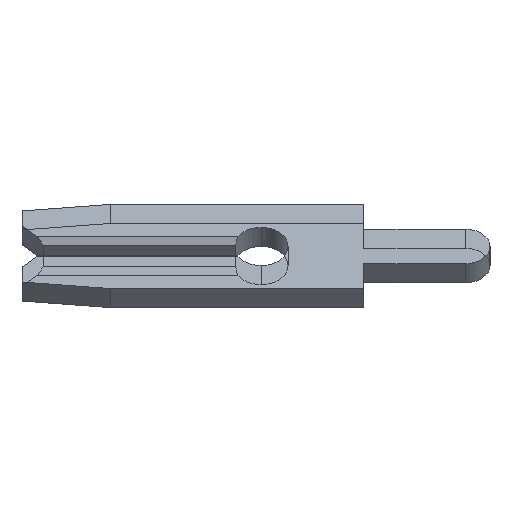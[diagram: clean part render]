
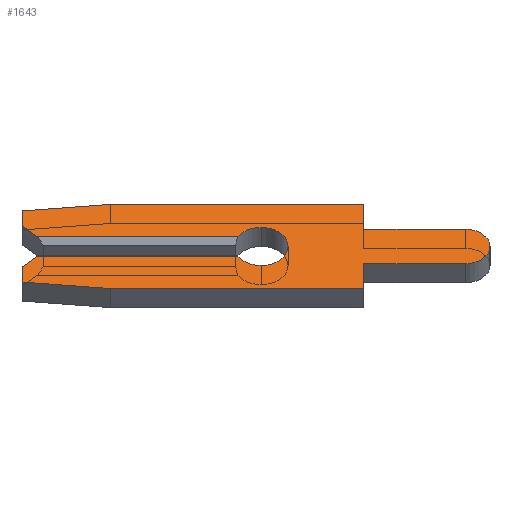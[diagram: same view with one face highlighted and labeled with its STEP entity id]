
A CAD part, left-side view. The second image highlights one B-rep face of the part: STEP entity #1643.
In plain terms, the highlighted face is planar.
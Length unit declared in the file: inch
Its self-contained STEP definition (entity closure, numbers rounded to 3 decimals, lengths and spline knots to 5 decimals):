
#25 = VERTEX_POINT ( 'NONE', #2202 ) ;
#42 = DIRECTION ( 'NONE',  ( 0., 0.995, 0.105 ) ) ;
#48 = CARTESIAN_POINT ( 'NONE',  ( -0.013, 0., 0. ) ) ;
#61 = LINE ( 'NONE', #1256, #2127 ) ;
#97 = FACE_OUTER_BOUND ( 'NONE', #2374, .T. ) ;
#131 = LINE ( 'NONE', #2694, #1034 ) ;
#137 = CARTESIAN_POINT ( 'NONE',  ( -0.013, 0.231, -0.028 ) ) ;
#149 = DIRECTION ( 'NONE',  ( 0., -1., 0. ) ) ;
#158 = CIRCLE ( 'NONE', #1631, 0.026 ) ;
#190 = VECTOR ( 'NONE', #2480, 39.37008 ) ;
#211 = DIRECTION ( 'NONE',  ( 0., 1., 0. ) ) ;
#214 = CARTESIAN_POINT ( 'NONE',  ( -0.013, 0.146, -0.0575 ) ) ;
#241 = DIRECTION ( 'NONE',  ( 0., 0., 1. ) ) ;
#283 = VERTEX_POINT ( 'NONE', #912 ) ;
#287 = ORIENTED_EDGE ( 'NONE', *, *, #1751, .T. ) ;
#288 = DIRECTION ( 'NONE',  ( -1., 0., 0. ) ) ;
#302 = VECTOR ( 'NONE', #211, 39.37008 ) ;
#349 = VERTEX_POINT ( 'NONE', #1965 ) ;
#353 = EDGE_CURVE ( 'NONE', #349, #859, #659, .T. ) ;
#354 = CARTESIAN_POINT ( 'NONE',  ( -0.013, 0.231, -0.04857 ) ) ;
#442 = VERTEX_POINT ( 'NONE', #2234 ) ;
#444 = ORIENTED_EDGE ( 'NONE', *, *, #353, .F. ) ;
#471 = AXIS2_PLACEMENT_3D ( 'NONE', #1158, #2653, #241 ) ;
#498 = DIRECTION ( 'NONE',  ( 0., 0., -1. ) ) ;
#543 = DIRECTION ( 'NONE',  ( 0., -0.707, 0.707 ) ) ;
#551 = LINE ( 'NONE', #764, #583 ) ;
#583 = VECTOR ( 'NONE', #543, 39.37008 ) ;
#588 = CARTESIAN_POINT ( 'NONE',  ( -0.013, -0.099, 0.0575 ) ) ;
#619 = VECTOR ( 'NONE', #1508, 39.37008 ) ;
#635 = DIRECTION ( 'NONE',  ( 0., 0., -1. ) ) ;
#645 = EDGE_CURVE ( 'NONE', #779, #1606, #2792, .T. ) ;
#659 = LINE ( 'NONE', #1589, #302 ) ;
#667 = LINE ( 'NONE', #137, #722 ) ;
#681 = EDGE_CURVE ( 'NONE', #1288, #2090, #131, .T. ) ;
#722 = VECTOR ( 'NONE', #1015, 39.37008 ) ;
#724 = ORIENTED_EDGE ( 'NONE', *, *, #2002, .F. ) ;
#764 = CARTESIAN_POINT ( 'NONE',  ( -0.013, 0.2105, -0.0075 ) ) ;
#769 = ORIENTED_EDGE ( 'NONE', *, *, #1484, .F. ) ;
#779 = VERTEX_POINT ( 'NONE', #214 ) ;
#782 = LINE ( 'NONE', #1839, #1663 ) ;
#784 = VECTOR ( 'NONE', #1238, 39.37008 ) ;
#800 = CARTESIAN_POINT ( 'NONE',  ( -0.013, 0.2105, 0.0075 ) ) ;
#839 = VERTEX_POINT ( 'NONE', #1217 ) ;
#841 = EDGE_CURVE ( 'NONE', #283, #2540, #1185, .T. ) ;
#859 = VERTEX_POINT ( 'NONE', #1626 ) ;
#865 = VERTEX_POINT ( 'NONE', #1412 ) ;
#892 = VECTOR ( 'NONE', #2773, 39.37008 ) ;
#912 = CARTESIAN_POINT ( 'NONE',  ( -0.013, 0.02252, -0.013 ) ) ;
#929 = LINE ( 'NONE', #2188, #1524 ) ;
#942 = ORIENTED_EDGE ( 'NONE', *, *, #1249, .F. ) ;
#1007 = CARTESIAN_POINT ( 'NONE',  ( -0.013, 0.146, 0.0575 ) ) ;
#1015 = DIRECTION ( 'NONE',  ( 0., 0., 1. ) ) ;
#1034 = VECTOR ( 'NONE', #1646, 39.37008 ) ;
#1036 = EDGE_CURVE ( 'NONE', #1885, #283, #2604, .T. ) ;
#1080 = ORIENTED_EDGE ( 'NONE', *, *, #645, .F. ) ;
#1108 = CIRCLE ( 'NONE', #1919, 0.026 ) ;
#1111 = VECTOR ( 'NONE', #42, 39.37008 ) ;
#1147 = LINE ( 'NONE', #1500, #619 ) ;
#1158 = CARTESIAN_POINT ( 'NONE',  ( -0.013, -0.1975, 0. ) ) ;
#1174 = CARTESIAN_POINT ( 'NONE',  ( -0.013, 0., 0. ) ) ;
#1185 = CIRCLE ( 'NONE', #1266, 0.026 ) ;
#1217 = CARTESIAN_POINT ( 'NONE',  ( -0.013, 0.146, 0.0575 ) ) ;
#1221 = LINE ( 'NONE', #1756, #190 ) ;
#1238 = DIRECTION ( 'NONE',  ( 0., -1., 0. ) ) ;
#1249 = EDGE_CURVE ( 'NONE', #865, #25, #1565, .T. ) ;
#1256 = CARTESIAN_POINT ( 'NONE',  ( -0.013, 0.146, -0.0575 ) ) ;
#1266 = AXIS2_PLACEMENT_3D ( 'NONE', #48, #288, #498 ) ;
#1288 = VERTEX_POINT ( 'NONE', #1461 ) ;
#1319 = VECTOR ( 'NONE', #2176, 39.37008 ) ;
#1341 = EDGE_CURVE ( 'NONE', #2473, #1885, #551, .T. ) ;
#1351 = ORIENTED_EDGE ( 'NONE', *, *, #1445, .F. ) ;
#1376 = CARTESIAN_POINT ( 'NONE',  ( -0.013, -0.1975, 0.0235 ) ) ;
#1398 = EDGE_CURVE ( 'NONE', #839, #2768, #2130, .T. ) ;
#1412 = CARTESIAN_POINT ( 'NONE',  ( -0.013, 0.231, 0.028 ) ) ;
#1423 = ORIENTED_EDGE ( 'NONE', *, *, #2588, .F. ) ;
#1445 = EDGE_CURVE ( 'NONE', #1606, #2473, #667, .T. ) ;
#1461 = CARTESIAN_POINT ( 'NONE',  ( -0.013, -0.099, 0.0235 ) ) ;
#1471 = ORIENTED_EDGE ( 'NONE', *, *, #2355, .F. ) ;
#1476 = CARTESIAN_POINT ( 'NONE',  ( -0.013, 0., 0. ) ) ;
#1484 = EDGE_CURVE ( 'NONE', #442, #779, #61, .T. ) ;
#1489 = CARTESIAN_POINT ( 'NONE',  ( -0.013, 0.02252, 0.013 ) ) ;
#1500 = CARTESIAN_POINT ( 'NONE',  ( -0.013, -0.099, -0.0575 ) ) ;
#1508 = DIRECTION ( 'NONE',  ( 0., 0., -1. ) ) ;
#1524 = VECTOR ( 'NONE', #149, 39.37008 ) ;
#1565 = LINE ( 'NONE', #2133, #2680 ) ;
#1589 = CARTESIAN_POINT ( 'NONE',  ( -0.013, -0.099, -0.0235 ) ) ;
#1603 = VERTEX_POINT ( 'NONE', #1489 ) ;
#1606 = VERTEX_POINT ( 'NONE', #354 ) ;
#1615 = CARTESIAN_POINT ( 'NONE',  ( -0.013, 0.231, -0.028 ) ) ;
#1622 = DIRECTION ( 'NONE',  ( 0., 0., -1. ) ) ;
#1626 = CARTESIAN_POINT ( 'NONE',  ( -0.013, -0.099, -0.0235 ) ) ;
#1631 = AXIS2_PLACEMENT_3D ( 'NONE', #1476, #2619, #2851 ) ;
#1635 = ORIENTED_EDGE ( 'NONE', *, *, #2047, .F. ) ;
#1638 = EDGE_CURVE ( 'NONE', #859, #442, #1147, .T. ) ;
#1643 = ADVANCED_FACE ( 'NONE', ( #97 ), #1949, .F. ) ;
#1646 = DIRECTION ( 'NONE',  ( 0., -1., 0. ) ) ;
#1663 = VECTOR ( 'NONE', #2432, 39.37008 ) ;
#1671 = ORIENTED_EDGE ( 'NONE', *, *, #1789, .F. ) ;
#1681 = DIRECTION ( 'NONE',  ( 0., 0., 1. ) ) ;
#1695 = DIRECTION ( 'NONE',  ( 0., 1., 0. ) ) ;
#1751 = EDGE_CURVE ( 'NONE', #2097, #1603, #929, .T. ) ;
#1756 = CARTESIAN_POINT ( 'NONE',  ( -0.013, -0.099, 0.0575 ) ) ;
#1759 = ORIENTED_EDGE ( 'NONE', *, *, #1992, .F. ) ;
#1789 = EDGE_CURVE ( 'NONE', #2031, #1603, #158, .T. ) ;
#1839 = CARTESIAN_POINT ( 'NONE',  ( -0.013, 0.231, 0.04857 ) ) ;
#1856 = ORIENTED_EDGE ( 'NONE', *, *, #1398, .F. ) ;
#1885 = VERTEX_POINT ( 'NONE', #2209 ) ;
#1919 = AXIS2_PLACEMENT_3D ( 'NONE', #1174, #2742, #1622 ) ;
#1949 = PLANE ( 'NONE',  #2478 ) ;
#1965 = CARTESIAN_POINT ( 'NONE',  ( -0.013, -0.1975, -0.0235 ) ) ;
#1972 = CARTESIAN_POINT ( 'NONE',  ( -0.013, 0., 0. ) ) ;
#1992 = EDGE_CURVE ( 'NONE', #25, #839, #782, .T. ) ;
#2002 = EDGE_CURVE ( 'NONE', #2768, #1288, #1221, .T. ) ;
#2028 = ORIENTED_EDGE ( 'NONE', *, *, #1341, .F. ) ;
#2031 = VERTEX_POINT ( 'NONE', #2037 ) ;
#2037 = CARTESIAN_POINT ( 'NONE',  ( -0.013, 0., 0.026 ) ) ;
#2047 = EDGE_CURVE ( 'NONE', #2090, #349, #2504, .T. ) ;
#2090 = VERTEX_POINT ( 'NONE', #1376 ) ;
#2097 = VERTEX_POINT ( 'NONE', #2639 ) ;
#2100 = ORIENTED_EDGE ( 'NONE', *, *, #681, .F. ) ;
#2127 = VECTOR ( 'NONE', #1695, 39.37008 ) ;
#2130 = LINE ( 'NONE', #1007, #892 ) ;
#2133 = CARTESIAN_POINT ( 'NONE',  ( -0.013, 0.231, 0.028 ) ) ;
#2147 = CARTESIAN_POINT ( 'NONE',  ( -0.013, 0., -0.013 ) ) ;
#2172 = DIRECTION ( 'NONE',  ( 1., 0., 0. ) ) ;
#2176 = DIRECTION ( 'NONE',  ( 0., 0.707, 0.707 ) ) ;
#2188 = CARTESIAN_POINT ( 'NONE',  ( -0.013, 0.231, 0.013 ) ) ;
#2191 = LINE ( 'NONE', #800, #1319 ) ;
#2202 = CARTESIAN_POINT ( 'NONE',  ( -0.013, 0.231, 0.04857 ) ) ;
#2209 = CARTESIAN_POINT ( 'NONE',  ( -0.013, 0.216, -0.013 ) ) ;
#2217 = ORIENTED_EDGE ( 'NONE', *, *, #841, .F. ) ;
#2234 = CARTESIAN_POINT ( 'NONE',  ( -0.013, -0.099, -0.0575 ) ) ;
#2355 = EDGE_CURVE ( 'NONE', #2540, #2031, #1108, .T. ) ;
#2374 = EDGE_LOOP ( 'NONE', ( #287, #1671, #1471, #2217, #2544, #2028, #1351, #1080, #769, #2467, #444, #1635, #2100, #724, #1856, #1759, #942, #1423 ) ) ;
#2432 = DIRECTION ( 'NONE',  ( 0., -0.995, 0.105 ) ) ;
#2467 = ORIENTED_EDGE ( 'NONE', *, *, #1638, .F. ) ;
#2470 = CARTESIAN_POINT ( 'NONE',  ( -0.013, 0.231, -0.04857 ) ) ;
#2473 = VERTEX_POINT ( 'NONE', #1615 ) ;
#2478 = AXIS2_PLACEMENT_3D ( 'NONE', #1972, #2172, #635 ) ;
#2480 = DIRECTION ( 'NONE',  ( 0., 0., -1. ) ) ;
#2504 = CIRCLE ( 'NONE', #471, 0.0235 ) ;
#2540 = VERTEX_POINT ( 'NONE', #2586 ) ;
#2544 = ORIENTED_EDGE ( 'NONE', *, *, #1036, .F. ) ;
#2586 = CARTESIAN_POINT ( 'NONE',  ( -0.013, 0., -0.026 ) ) ;
#2588 = EDGE_CURVE ( 'NONE', #2097, #865, #2191, .T. ) ;
#2604 = LINE ( 'NONE', #2147, #784 ) ;
#2619 = DIRECTION ( 'NONE',  ( -1., 0., 0. ) ) ;
#2639 = CARTESIAN_POINT ( 'NONE',  ( -0.013, 0.216, 0.013 ) ) ;
#2653 = DIRECTION ( 'NONE',  ( 1., 0., 0. ) ) ;
#2680 = VECTOR ( 'NONE', #1681, 39.37008 ) ;
#2694 = CARTESIAN_POINT ( 'NONE',  ( -0.013, -0.099, 0.0235 ) ) ;
#2742 = DIRECTION ( 'NONE',  ( -1., 0., 0. ) ) ;
#2768 = VERTEX_POINT ( 'NONE', #588 ) ;
#2773 = DIRECTION ( 'NONE',  ( 0., -1., 0. ) ) ;
#2792 = LINE ( 'NONE', #2470, #1111 ) ;
#2851 = DIRECTION ( 'NONE',  ( 0., 0., -1. ) ) ;
